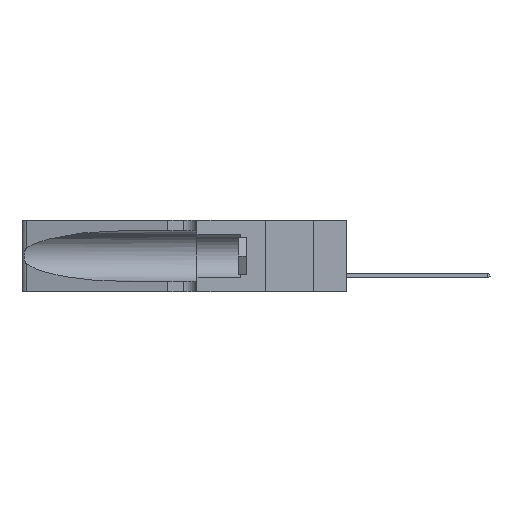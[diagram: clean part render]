
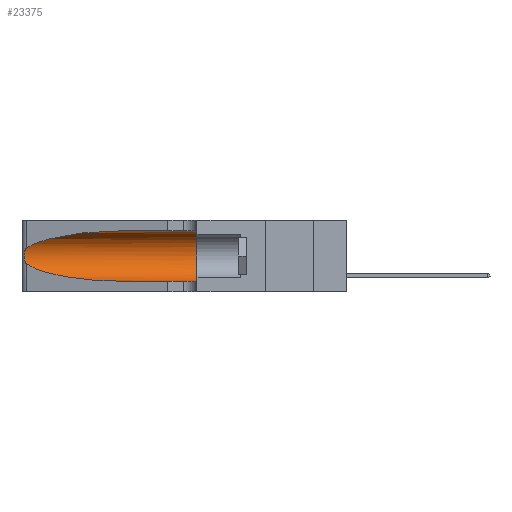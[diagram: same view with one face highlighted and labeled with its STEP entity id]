
A CAD part, left-side view. The second image highlights one B-rep face of the part: STEP entity #23375.
In plain terms, the highlighted cylindrical face has radius 3.308 mm (diameter 6.617 mm), a partial arc.
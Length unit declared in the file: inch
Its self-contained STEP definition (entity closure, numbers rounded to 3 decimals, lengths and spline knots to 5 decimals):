
#1786 = EDGE_CURVE ( 'NONE', #12944, #18891, #6484, .T. ) ;
#1930 = DIRECTION ( 'NONE',  ( 0., -1., 0. ) ) ;
#3604 = ORIENTED_EDGE ( 'NONE', *, *, #1786, .F. ) ;
#3782 = DIRECTION ( 'NONE',  ( 0., -1., 0. ) ) ;
#4564 = B_SPLINE_CURVE_WITH_KNOTS ( 'NONE', 3,
 ( #7161, #20404, #9063, #22302, #22049, #22375, #22132, #10955, #11034, #10718, #24221, #18555, #12626, #24312 ),
 .UNSPECIFIED., .F., .F.,
 ( 4, 2, 2, 2, 2, 2, 4 ),
 ( 0., 0.00027, 0.00053, 0.00107, 0.0016, 0.00187, 0.00214 ),
 .UNSPECIFIED. ) ;
#5610 = ORIENTED_EDGE ( 'NONE', *, *, #5791, .T. ) ;
#5748 = CARTESIAN_POINT ( 'NONE',  ( 0.1305, 0.35, 0.185 ) ) ;
#5790 = CARTESIAN_POINT ( 'NONE',  ( 0.1305, 1.61858, 0.05475 ) ) ;
#5791 = EDGE_CURVE ( 'NONE', #9532, #15445, #4564, .T. ) ;
#6059 = EDGE_LOOP ( 'NONE', ( #24166, #5610, #17590, #6503, #21956, #3604 ) ) ;
#6469 = CARTESIAN_POINT ( 'NONE',  ( 0.25487, 1.22718, 0.14631 ) ) ;
#6484 = LINE ( 'NONE', #11420, #16537 ) ;
#6503 = ORIENTED_EDGE ( 'NONE', *, *, #14706, .T. ) ;
#6509 = VECTOR ( 'NONE', #3782, 39.37008 ) ;
#7161 = CARTESIAN_POINT ( 'NONE',  ( 0.25487, 1.22718, 0.22369 ) ) ;
#7184 =( BOUNDED_CURVE ( )  B_SPLINE_CURVE ( 3, ( #16437, #12509, #24502, #18502 ),
 .UNSPECIFIED., .F., .F. ) 
 B_SPLINE_CURVE_WITH_KNOTS ( ( 4, 4 ),
 ( 1.5708, 2.84003 ),
 .UNSPECIFIED. ) 
 CURVE ( )  GEOMETRIC_REPRESENTATION_ITEM ( )  RATIONAL_B_SPLINE_CURVE ( ( 1., 0.87, 0.87, 1. ) ) 
 REPRESENTATION_ITEM ( '' )  );
#7533 = DIRECTION ( 'NONE',  ( 0., 0., -1. ) ) ;
#7684 = DIRECTION ( 'NONE',  ( 0., 1., 0. ) ) ;
#9063 = CARTESIAN_POINT ( 'NONE',  ( 0.25639, 1.23184, 0.21858 ) ) ;
#9532 = VERTEX_POINT ( 'NONE', #18358 ) ;
#10459 = CARTESIAN_POINT ( 'NONE',  ( 0.1305, 0.35, 0.31525 ) ) ;
#10718 = CARTESIAN_POINT ( 'NONE',  ( 0.25856, 1.23593, 0.16098 ) ) ;
#10955 = CARTESIAN_POINT ( 'NONE',  ( 0.26075, 1.23896, 0.178 ) ) ;
#11034 = CARTESIAN_POINT ( 'NONE',  ( 0.26017, 1.23833, 0.17102 ) ) ;
#11420 = CARTESIAN_POINT ( 'NONE',  ( 0.1305, 1.61858, 0.31525 ) ) ;
#11586 =( BOUNDED_CURVE ( )  B_SPLINE_CURVE ( 3, ( #6469, #21368, #15808, #21615 ),
 .UNSPECIFIED., .F., .F. ) 
 B_SPLINE_CURVE_WITH_KNOTS ( ( 4, 4 ),
 ( 3.44316, 4.71239 ),
 .UNSPECIFIED. ) 
 CURVE ( )  GEOMETRIC_REPRESENTATION_ITEM ( )  RATIONAL_B_SPLINE_CURVE ( ( 1., 0.87, 0.87, 1. ) ) 
 REPRESENTATION_ITEM ( '' )  );
#11914 = CARTESIAN_POINT ( 'NONE',  ( 0.1305, 0.35, 0.05475 ) ) ;
#12420 = VERTEX_POINT ( 'NONE', #14851 ) ;
#12509 = CARTESIAN_POINT ( 'NONE',  ( 0.18966, 0.96281, 0.31525 ) ) ;
#12626 = CARTESIAN_POINT ( 'NONE',  ( 0.25555, 1.22993, 0.14849 ) ) ;
#12745 = LINE ( 'NONE', #5790, #6509 ) ;
#12944 = VERTEX_POINT ( 'NONE', #23974 ) ;
#13341 = CIRCLE ( 'NONE', #19392, 0.13025 ) ;
#13823 = FACE_OUTER_BOUND ( 'NONE', #6059, .T. ) ;
#14706 = EDGE_CURVE ( 'NONE', #12420, #23863, #12745, .T. ) ;
#14851 = CARTESIAN_POINT ( 'NONE',  ( 0.1305, 0.72297, 0.05475 ) ) ;
#15053 = CARTESIAN_POINT ( 'NONE',  ( 0.1305, 1.61858, 0.185 ) ) ;
#15445 = VERTEX_POINT ( 'NONE', #21414 ) ;
#15808 = CARTESIAN_POINT ( 'NONE',  ( 0.18966, 0.96281, 0.05475 ) ) ;
#16437 = CARTESIAN_POINT ( 'NONE',  ( 0.1305, 0.72297, 0.31525 ) ) ;
#16537 = VECTOR ( 'NONE', #1930, 39.37008 ) ;
#17112 = EDGE_CURVE ( 'NONE', #15445, #12420, #11586, .T. ) ;
#17590 = ORIENTED_EDGE ( 'NONE', *, *, #17112, .T. ) ;
#17652 = CYLINDRICAL_SURFACE ( 'NONE', #24384, 0.13025 ) ;
#18358 = CARTESIAN_POINT ( 'NONE',  ( 0.25487, 1.22718, 0.22369 ) ) ;
#18502 = CARTESIAN_POINT ( 'NONE',  ( 0.25487, 1.22718, 0.22369 ) ) ;
#18555 = CARTESIAN_POINT ( 'NONE',  ( 0.25639, 1.23186, 0.15144 ) ) ;
#18861 = DIRECTION ( 'NONE',  ( 0., -1., 0. ) ) ;
#18891 = VERTEX_POINT ( 'NONE', #10459 ) ;
#19392 = AXIS2_PLACEMENT_3D ( 'NONE', #5748, #7684, #20905 ) ;
#19759 = EDGE_CURVE ( 'NONE', #12944, #9532, #7184, .T. ) ;
#20404 = CARTESIAN_POINT ( 'NONE',  ( 0.25555, 1.22994, 0.2215 ) ) ;
#20708 = EDGE_CURVE ( 'NONE', #18891, #23863, #13341, .T. ) ;
#20905 = DIRECTION ( 'NONE',  ( 0., 0., 1. ) ) ;
#21368 = CARTESIAN_POINT ( 'NONE',  ( 0.2373, 1.15595, 0.08982 ) ) ;
#21414 = CARTESIAN_POINT ( 'NONE',  ( 0.25487, 1.22718, 0.14631 ) ) ;
#21615 = CARTESIAN_POINT ( 'NONE',  ( 0.1305, 0.72297, 0.05475 ) ) ;
#21956 = ORIENTED_EDGE ( 'NONE', *, *, #20708, .F. ) ;
#22049 = CARTESIAN_POINT ( 'NONE',  ( 0.25854, 1.2359, 0.20912 ) ) ;
#22132 = CARTESIAN_POINT ( 'NONE',  ( 0.26075, 1.23896, 0.19203 ) ) ;
#22302 = CARTESIAN_POINT ( 'NONE',  ( 0.25787, 1.23484, 0.2124 ) ) ;
#22375 = CARTESIAN_POINT ( 'NONE',  ( 0.26018, 1.23835, 0.19895 ) ) ;
#23375 = ADVANCED_FACE ( 'NONE', ( #13823 ), #17652, .F. ) ;
#23863 = VERTEX_POINT ( 'NONE', #11914 ) ;
#23974 = CARTESIAN_POINT ( 'NONE',  ( 0.1305, 0.72297, 0.31525 ) ) ;
#24166 = ORIENTED_EDGE ( 'NONE', *, *, #19759, .T. ) ;
#24221 = CARTESIAN_POINT ( 'NONE',  ( 0.25789, 1.23486, 0.15765 ) ) ;
#24312 = CARTESIAN_POINT ( 'NONE',  ( 0.25487, 1.22718, 0.14631 ) ) ;
#24384 = AXIS2_PLACEMENT_3D ( 'NONE', #15053, #18861, #7533 ) ;
#24502 = CARTESIAN_POINT ( 'NONE',  ( 0.2373, 1.15595, 0.28018 ) ) ;
